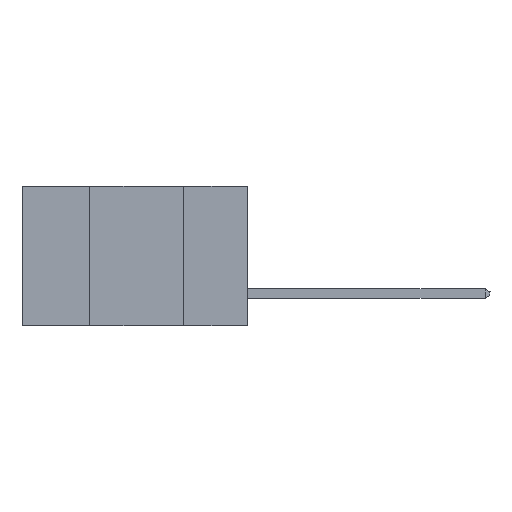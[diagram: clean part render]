
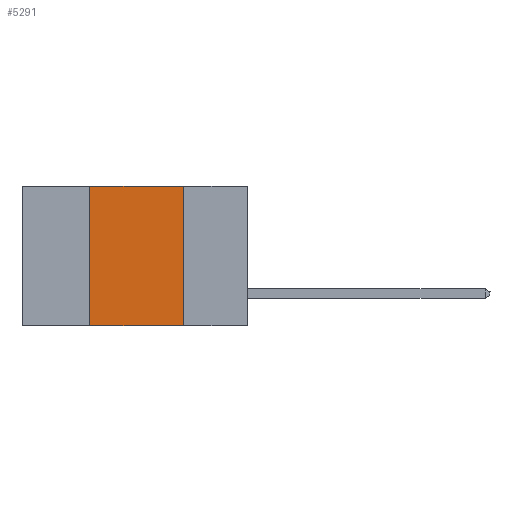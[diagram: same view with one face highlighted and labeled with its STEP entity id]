
A CAD part, left-side view. The second image highlights one B-rep face of the part: STEP entity #5291.
In plain terms, the highlighted planar face has unit normal (-1, 0, 0).
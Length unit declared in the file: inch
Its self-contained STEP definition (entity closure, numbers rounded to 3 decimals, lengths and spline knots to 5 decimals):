
#216 = EDGE_CURVE ( 'NONE', #2246, #7751, #3046, .T. ) ;
#563 = DIRECTION ( 'NONE',  ( 0., 0., -1. ) ) ;
#686 = CARTESIAN_POINT ( 'NONE',  ( 0., 0.17, 0. ) ) ;
#902 = DIRECTION ( 'NONE',  ( 0., -1., 0. ) ) ;
#1120 = DIRECTION ( 'NONE',  ( 0., 0., -1. ) ) ;
#1400 = CARTESIAN_POINT ( 'NONE',  ( 0., 0.6, 0. ) ) ;
#1609 = ORIENTED_EDGE ( 'NONE', *, *, #216, .F. ) ;
#1913 = EDGE_LOOP ( 'NONE', ( #4746, #10193, #1609, #6159 ) ) ;
#1969 = EDGE_CURVE ( 'NONE', #7751, #4233, #9616, .T. ) ;
#2204 = PLANE ( 'NONE',  #9579 ) ;
#2229 = VERTEX_POINT ( 'NONE', #5741 ) ;
#2246 = VERTEX_POINT ( 'NONE', #3939 ) ;
#3046 = LINE ( 'NONE', #5738, #5734 ) ;
#3363 = VECTOR ( 'NONE', #5900, 39.37008 ) ;
#3694 = DIRECTION ( 'NONE',  ( 0., 0., 1. ) ) ;
#3785 = VECTOR ( 'NONE', #902, 39.37008 ) ;
#3939 = CARTESIAN_POINT ( 'NONE',  ( 0., 0.42, -0.37 ) ) ;
#4233 = VERTEX_POINT ( 'NONE', #686 ) ;
#4746 = ORIENTED_EDGE ( 'NONE', *, *, #8839, .F. ) ;
#4852 = DIRECTION ( 'NONE',  ( 1., 0., 0. ) ) ;
#5291 = ADVANCED_FACE ( 'NONE', ( #7626 ), #2204, .F. ) ;
#5488 = CARTESIAN_POINT ( 'NONE',  ( 0., 0.6, -0.37 ) ) ;
#5734 = VECTOR ( 'NONE', #3694, 39.37008 ) ;
#5738 = CARTESIAN_POINT ( 'NONE',  ( 0., 0.42, -0.37 ) ) ;
#5741 = CARTESIAN_POINT ( 'NONE',  ( 0., 0.17, -0.37 ) ) ;
#5900 = DIRECTION ( 'NONE',  ( 0., -1., 0. ) ) ;
#6159 = ORIENTED_EDGE ( 'NONE', *, *, #10377, .T. ) ;
#6764 = LINE ( 'NONE', #8808, #11819 ) ;
#7626 = FACE_OUTER_BOUND ( 'NONE', #1913, .T. ) ;
#7751 = VERTEX_POINT ( 'NONE', #10652 ) ;
#8399 = CARTESIAN_POINT ( 'NONE',  ( 0., 0.6, 0. ) ) ;
#8808 = CARTESIAN_POINT ( 'NONE',  ( 0., 0.17, -0.37 ) ) ;
#8839 = EDGE_CURVE ( 'NONE', #4233, #2229, #6764, .T. ) ;
#9244 = LINE ( 'NONE', #5488, #3785 ) ;
#9579 = AXIS2_PLACEMENT_3D ( 'NONE', #8399, #4852, #1120 ) ;
#9616 = LINE ( 'NONE', #1400, #3363 ) ;
#10193 = ORIENTED_EDGE ( 'NONE', *, *, #1969, .F. ) ;
#10377 = EDGE_CURVE ( 'NONE', #2246, #2229, #9244, .T. ) ;
#10652 = CARTESIAN_POINT ( 'NONE',  ( 0., 0.42, 0. ) ) ;
#11819 = VECTOR ( 'NONE', #563, 39.37008 ) ;
